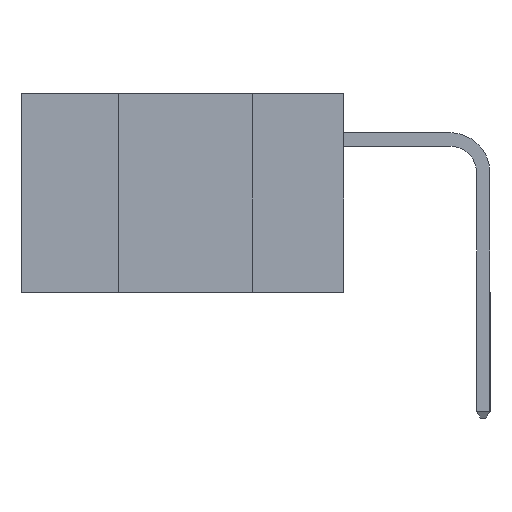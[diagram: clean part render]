
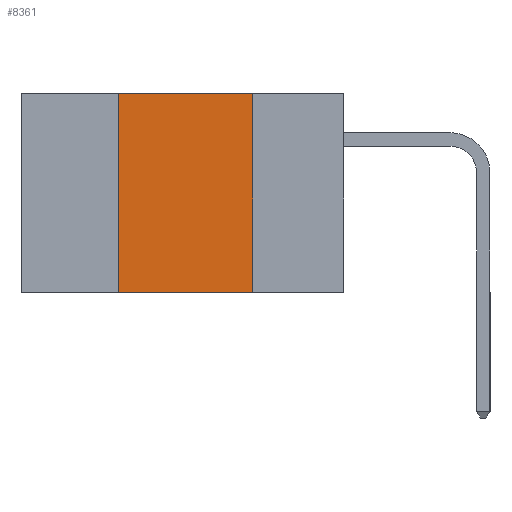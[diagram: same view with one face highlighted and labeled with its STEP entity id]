
A CAD part, left-side view. The second image highlights one B-rep face of the part: STEP entity #8361.
In plain terms, the highlighted planar face has unit normal (-1, 0, 0).
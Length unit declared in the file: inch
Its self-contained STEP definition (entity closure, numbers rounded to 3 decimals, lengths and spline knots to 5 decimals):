
#717 = VERTEX_POINT ( 'NONE', #6155 ) ;
#1039 = VERTEX_POINT ( 'NONE', #10840 ) ;
#2208 = DIRECTION ( 'NONE',  ( 1., 0., 0. ) ) ;
#3582 = CARTESIAN_POINT ( 'NONE',  ( 0., 0.17, -0.37 ) ) ;
#3942 = EDGE_LOOP ( 'NONE', ( #5687, #17383, #4986, #11719 ) ) ;
#4301 = DIRECTION ( 'NONE',  ( 0., -1., 0. ) ) ;
#4656 = LINE ( 'NONE', #16182, #7392 ) ;
#4986 = ORIENTED_EDGE ( 'NONE', *, *, #18883, .F. ) ;
#5362 = CARTESIAN_POINT ( 'NONE',  ( 0., 0.6, 0. ) ) ;
#5403 = LINE ( 'NONE', #18199, #18018 ) ;
#5687 = ORIENTED_EDGE ( 'NONE', *, *, #19253, .F. ) ;
#6155 = CARTESIAN_POINT ( 'NONE',  ( 0., 0.17, 0. ) ) ;
#6163 = EDGE_CURVE ( 'NONE', #1039, #14451, #5403, .T. ) ;
#6288 = AXIS2_PLACEMENT_3D ( 'NONE', #5362, #2208, #9670 ) ;
#7392 = VECTOR ( 'NONE', #19298, 39.37008 ) ;
#8361 = ADVANCED_FACE ( 'NONE', ( #10689 ), #12896, .F. ) ;
#8590 = CARTESIAN_POINT ( 'NONE',  ( 0., 0.17, 0. ) ) ;
#9165 = LINE ( 'NONE', #8590, #12377 ) ;
#9670 = DIRECTION ( 'NONE',  ( 0., 0., -1. ) ) ;
#10181 = CARTESIAN_POINT ( 'NONE',  ( 0., 0.42, 0. ) ) ;
#10200 = DIRECTION ( 'NONE',  ( 0., 0., -1. ) ) ;
#10689 = FACE_OUTER_BOUND ( 'NONE', #3942, .T. ) ;
#10840 = CARTESIAN_POINT ( 'NONE',  ( 0., 0.42, -0.37 ) ) ;
#11428 = VECTOR ( 'NONE', #12408, 39.37008 ) ;
#11719 = ORIENTED_EDGE ( 'NONE', *, *, #6163, .T. ) ;
#12377 = VECTOR ( 'NONE', #10200, 39.37008 ) ;
#12408 = DIRECTION ( 'NONE',  ( 0., 0., 1. ) ) ;
#12896 = PLANE ( 'NONE',  #6288 ) ;
#13760 = EDGE_CURVE ( 'NONE', #18114, #717, #4656, .T. ) ;
#14451 = VERTEX_POINT ( 'NONE', #3582 ) ;
#16182 = CARTESIAN_POINT ( 'NONE',  ( 0., 0.6, 0. ) ) ;
#17383 = ORIENTED_EDGE ( 'NONE', *, *, #13760, .F. ) ;
#18018 = VECTOR ( 'NONE', #4301, 39.37008 ) ;
#18114 = VERTEX_POINT ( 'NONE', #10181 ) ;
#18199 = CARTESIAN_POINT ( 'NONE',  ( 0., 0.6, -0.37 ) ) ;
#18883 = EDGE_CURVE ( 'NONE', #1039, #18114, #20233, .T. ) ;
#19253 = EDGE_CURVE ( 'NONE', #717, #14451, #9165, .T. ) ;
#19298 = DIRECTION ( 'NONE',  ( 0., -1., 0. ) ) ;
#20200 = CARTESIAN_POINT ( 'NONE',  ( 0., 0.42, 0. ) ) ;
#20233 = LINE ( 'NONE', #20200, #11428 ) ;
